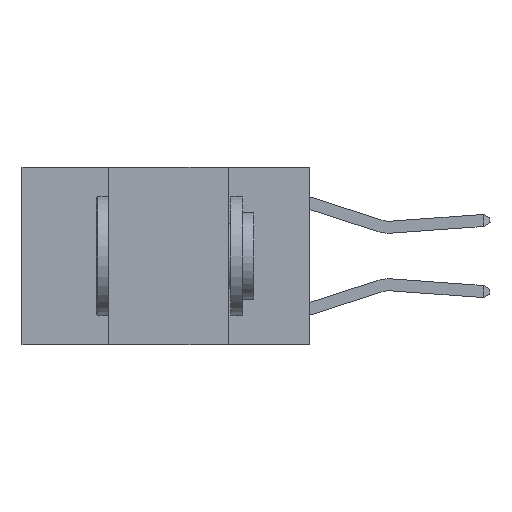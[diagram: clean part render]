
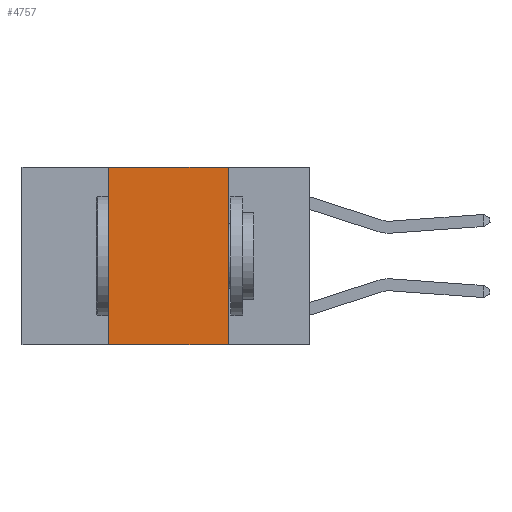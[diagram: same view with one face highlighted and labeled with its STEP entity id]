
A CAD part, left-side view. The second image highlights one B-rep face of the part: STEP entity #4757.
In plain terms, the highlighted planar face has unit normal (-1, 0, 0).
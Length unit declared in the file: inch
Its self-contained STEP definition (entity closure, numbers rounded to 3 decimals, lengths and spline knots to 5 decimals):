
#207 = EDGE_CURVE ( 'NONE', #10204, #4233, #3910, .T. ) ;
#1030 = CARTESIAN_POINT ( 'NONE',  ( 0., 0.17, -0.37 ) ) ;
#1298 = DIRECTION ( 'NONE',  ( 0., 0., -1. ) ) ;
#1386 = PLANE ( 'NONE',  #12694 ) ;
#1392 = LINE ( 'NONE', #15849, #14341 ) ;
#2313 = ORIENTED_EDGE ( 'NONE', *, *, #8789, .F. ) ;
#2580 = CARTESIAN_POINT ( 'NONE',  ( 0., 0.42, 0. ) ) ;
#2814 = ORIENTED_EDGE ( 'NONE', *, *, #207, .F. ) ;
#2852 = ORIENTED_EDGE ( 'NONE', *, *, #14860, .F. ) ;
#3240 = ORIENTED_EDGE ( 'NONE', *, *, #12044, .T. ) ;
#3283 = VERTEX_POINT ( 'NONE', #12349 ) ;
#3492 = LINE ( 'NONE', #10184, #9683 ) ;
#3910 = LINE ( 'NONE', #5410, #10085 ) ;
#4093 = DIRECTION ( 'NONE',  ( 1., 0., 0. ) ) ;
#4214 = FACE_OUTER_BOUND ( 'NONE', #10155, .T. ) ;
#4233 = VERTEX_POINT ( 'NONE', #11675 ) ;
#4757 = ADVANCED_FACE ( 'NONE', ( #4214 ), #1386, .F. ) ;
#4834 = DIRECTION ( 'NONE',  ( 0., -1., 0. ) ) ;
#5032 = VECTOR ( 'NONE', #10070, 39.37008 ) ;
#5410 = CARTESIAN_POINT ( 'NONE',  ( 0., 0.6, 0. ) ) ;
#6232 = DIRECTION ( 'NONE',  ( 0., -1., 0. ) ) ;
#7502 = LINE ( 'NONE', #2580, #5032 ) ;
#8789 = EDGE_CURVE ( 'NONE', #4233, #13097, #3492, .T. ) ;
#9683 = VECTOR ( 'NONE', #1298, 39.37008 ) ;
#10070 = DIRECTION ( 'NONE',  ( 0., 0., 1. ) ) ;
#10085 = VECTOR ( 'NONE', #6232, 39.37008 ) ;
#10155 = EDGE_LOOP ( 'NONE', ( #2313, #2814, #2852, #3240 ) ) ;
#10184 = CARTESIAN_POINT ( 'NONE',  ( 0., 0.17, 0. ) ) ;
#10204 = VERTEX_POINT ( 'NONE', #10326 ) ;
#10326 = CARTESIAN_POINT ( 'NONE',  ( 0., 0.42, 0. ) ) ;
#11675 = CARTESIAN_POINT ( 'NONE',  ( 0., 0.17, 0. ) ) ;
#12044 = EDGE_CURVE ( 'NONE', #3283, #13097, #1392, .T. ) ;
#12349 = CARTESIAN_POINT ( 'NONE',  ( 0., 0.42, -0.37 ) ) ;
#12694 = AXIS2_PLACEMENT_3D ( 'NONE', #15072, #4093, #12740 ) ;
#12740 = DIRECTION ( 'NONE',  ( 0., 0., -1. ) ) ;
#13097 = VERTEX_POINT ( 'NONE', #1030 ) ;
#14341 = VECTOR ( 'NONE', #4834, 39.37008 ) ;
#14860 = EDGE_CURVE ( 'NONE', #3283, #10204, #7502, .T. ) ;
#15072 = CARTESIAN_POINT ( 'NONE',  ( 0., 0.6, 0. ) ) ;
#15849 = CARTESIAN_POINT ( 'NONE',  ( 0., 0.6, -0.37 ) ) ;
